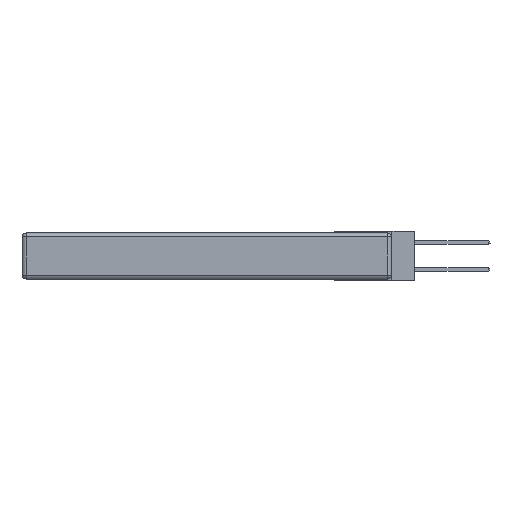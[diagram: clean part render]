
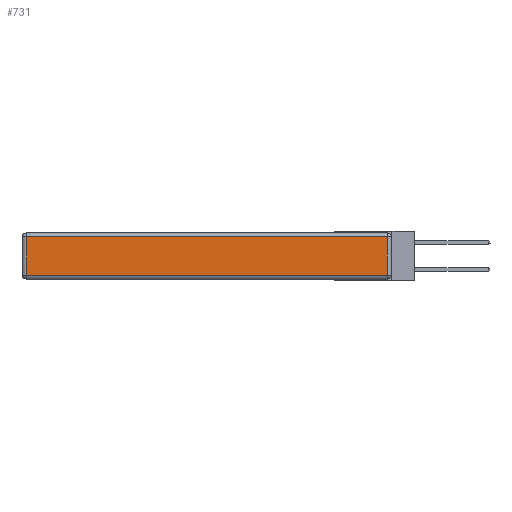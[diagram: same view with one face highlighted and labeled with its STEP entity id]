
A CAD part, left-side view. The second image highlights one B-rep face of the part: STEP entity #731.
In plain terms, the highlighted planar face has unit normal (-1, 0, 0).
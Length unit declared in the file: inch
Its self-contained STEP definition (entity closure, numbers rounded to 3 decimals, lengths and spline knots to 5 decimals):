
#110 = DIRECTION ( 'NONE',  ( 0., -1., 0. ) ) ;
#207 = EDGE_CURVE ( 'NONE', #16632, #26349, #13605, .T. ) ;
#731 = ADVANCED_FACE ( 'NONE', ( #1466 ), #2489, .T. ) ;
#1466 = FACE_OUTER_BOUND ( 'NONE', #15701, .T. ) ;
#2489 = PLANE ( 'NONE',  #23896 ) ;
#2793 = VERTEX_POINT ( 'NONE', #15251 ) ;
#2856 = DIRECTION ( 'NONE',  ( 0., 0., 1. ) ) ;
#5021 = LINE ( 'NONE', #8401, #19086 ) ;
#8401 = CARTESIAN_POINT ( 'NONE',  ( 0., 0., -0.313 ) ) ;
#8801 = DIRECTION ( 'NONE',  ( -1., 0., 0. ) ) ;
#9395 = DIRECTION ( 'NONE',  ( 0., 0., -1. ) ) ;
#9558 = ORIENTED_EDGE ( 'NONE', *, *, #10183, .T. ) ;
#10183 = EDGE_CURVE ( 'NONE', #2793, #16632, #26050, .T. ) ;
#11365 = CARTESIAN_POINT ( 'NONE',  ( 0., 0.03, -0.343 ) ) ;
#12949 = VECTOR ( 'NONE', #2856, 39.37008 ) ;
#13229 = VERTEX_POINT ( 'NONE', #15522 ) ;
#13605 = LINE ( 'NONE', #20015, #13931 ) ;
#13931 = VECTOR ( 'NONE', #9395, 39.37008 ) ;
#15251 = CARTESIAN_POINT ( 'NONE',  ( 0., 0.03, -0.03 ) ) ;
#15522 = CARTESIAN_POINT ( 'NONE',  ( 0., 0.03, -0.313 ) ) ;
#15607 = ORIENTED_EDGE ( 'NONE', *, *, #24140, .T. ) ;
#15701 = EDGE_LOOP ( 'NONE', ( #15607, #26607, #9558, #21525 ) ) ;
#15822 = VECTOR ( 'NONE', #26701, 39.37008 ) ;
#16131 = CARTESIAN_POINT ( 'NONE',  ( 0., 2.75, -0.03 ) ) ;
#16632 = VERTEX_POINT ( 'NONE', #19113 ) ;
#16906 = CARTESIAN_POINT ( 'NONE',  ( 0., 2.72, -0.313 ) ) ;
#19086 = VECTOR ( 'NONE', #110, 39.37008 ) ;
#19113 = CARTESIAN_POINT ( 'NONE',  ( 0., 2.72, -0.03 ) ) ;
#20015 = CARTESIAN_POINT ( 'NONE',  ( 0., 2.72, -0.343 ) ) ;
#21370 = CARTESIAN_POINT ( 'NONE',  ( 0., 0., -0.343 ) ) ;
#21525 = ORIENTED_EDGE ( 'NONE', *, *, #207, .T. ) ;
#22782 = LINE ( 'NONE', #11365, #12949 ) ;
#23483 = DIRECTION ( 'NONE',  ( 0., 0., 1. ) ) ;
#23896 = AXIS2_PLACEMENT_3D ( 'NONE', #21370, #8801, #23483 ) ;
#24140 = EDGE_CURVE ( 'NONE', #26349, #13229, #5021, .T. ) ;
#26045 = EDGE_CURVE ( 'NONE', #13229, #2793, #22782, .T. ) ;
#26050 = LINE ( 'NONE', #16131, #15822 ) ;
#26349 = VERTEX_POINT ( 'NONE', #16906 ) ;
#26607 = ORIENTED_EDGE ( 'NONE', *, *, #26045, .T. ) ;
#26701 = DIRECTION ( 'NONE',  ( 0., 1., 0. ) ) ;
